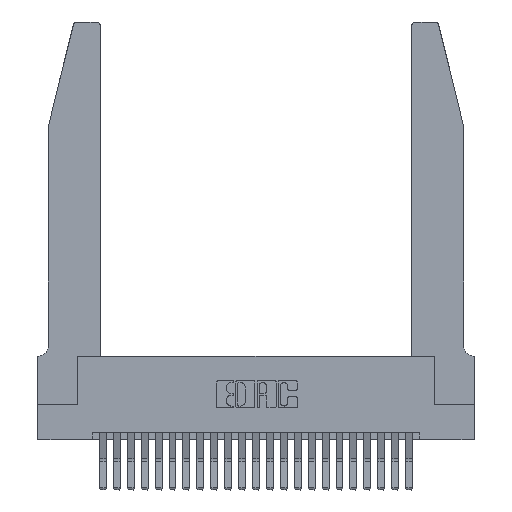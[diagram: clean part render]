
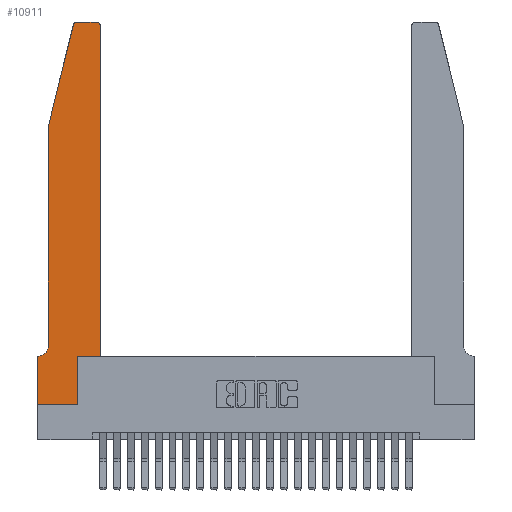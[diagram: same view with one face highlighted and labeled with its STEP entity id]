
A CAD part, top view. The second image highlights one B-rep face of the part: STEP entity #10911.
In plain terms, the highlighted planar face has unit normal (0, 0, 1).
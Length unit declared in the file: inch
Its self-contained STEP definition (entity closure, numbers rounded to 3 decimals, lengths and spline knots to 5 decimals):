
#15 = VECTOR ( 'NONE', #15309, 39.37008 ) ;
#550 = CARTESIAN_POINT ( 'NONE',  ( 0., 0., 0.37 ) ) ;
#933 = CARTESIAN_POINT ( 'NONE',  ( 0.0055, 0.35, 0.37 ) ) ;
#1262 = EDGE_CURVE ( 'NONE', #23223, #23100, #10198, .T. ) ;
#1471 = EDGE_LOOP ( 'NONE', ( #11044, #24769, #20503, #25360, #15903, #8886, #11153, #18814, #14873, #16694, #4052, #3981 ) ) ;
#1908 = EDGE_CURVE ( 'NONE', #11073, #17594, #23082, .T. ) ;
#2153 = VERTEX_POINT ( 'NONE', #11108 ) ;
#2604 = CARTESIAN_POINT ( 'NONE',  ( 0.284, 2.75, 0.37 ) ) ;
#2974 = VECTOR ( 'NONE', #14906, 39.37008 ) ;
#3108 = CARTESIAN_POINT ( 'NONE',  ( 0.0055, 0.42, 0.37 ) ) ;
#3163 = EDGE_CURVE ( 'NONE', #10190, #9971, #12925, .T. ) ;
#3170 = CIRCLE ( 'NONE', #18161, 0.03 ) ;
#3363 = CARTESIAN_POINT ( 'NONE',  ( 0.2865, 0.35, 0.37 ) ) ;
#3608 = EDGE_CURVE ( 'NONE', #23711, #13043, #4282, .T. ) ;
#3981 = ORIENTED_EDGE ( 'NONE', *, *, #11979, .T. ) ;
#4021 = DIRECTION ( 'NONE',  ( 0., -1., 0. ) ) ;
#4052 = ORIENTED_EDGE ( 'NONE', *, *, #1262, .T. ) ;
#4282 = LINE ( 'NONE', #23813, #11672 ) ;
#4654 = DIRECTION ( 'NONE',  ( 1., 0., 0. ) ) ;
#4776 = LINE ( 'NONE', #5056, #5112 ) ;
#4960 = CARTESIAN_POINT ( 'NONE',  ( 0.0755, 2., 0.37 ) ) ;
#5056 = CARTESIAN_POINT ( 'NONE',  ( 0.0755, 2., 0.37 ) ) ;
#5112 = VECTOR ( 'NONE', #18942, 39.37008 ) ;
#5397 = CARTESIAN_POINT ( 'NONE',  ( 0.284, 2.72, 0.37 ) ) ;
#5557 = CARTESIAN_POINT ( 'NONE',  ( 0., 0.35, 0.37 ) ) ;
#5687 = DIRECTION ( 'NONE',  ( 0., 1., 0. ) ) ;
#6547 = CARTESIAN_POINT ( 'NONE',  ( 0.4205, 2.72, 0.37 ) ) ;
#7175 = DIRECTION ( 'NONE',  ( 1., 0., 0. ) ) ;
#7464 = VECTOR ( 'NONE', #9497, 39.37008 ) ;
#8459 = DIRECTION ( 'NONE',  ( 1., 0., 0. ) ) ;
#8886 = ORIENTED_EDGE ( 'NONE', *, *, #1908, .T. ) ;
#9270 = DIRECTION ( 'NONE',  ( 0., 0., 1. ) ) ;
#9497 = DIRECTION ( 'NONE',  ( -1., 0., 0. ) ) ;
#9725 = CARTESIAN_POINT ( 'NONE',  ( 0.2865, 0.35, 0.37 ) ) ;
#9971 = VERTEX_POINT ( 'NONE', #2604 ) ;
#10190 = VERTEX_POINT ( 'NONE', #12941 ) ;
#10198 = LINE ( 'NONE', #10573, #15727 ) ;
#10573 = CARTESIAN_POINT ( 'NONE',  ( 0.4505, 0.35, 0.37 ) ) ;
#10820 = CARTESIAN_POINT ( 'NONE',  ( 0.4505, 0.35, 0.37 ) ) ;
#10904 = PLANE ( 'NONE',  #17168 ) ;
#10911 = ADVANCED_FACE ( 'NONE', ( #11515 ), #10904, .T. ) ;
#11044 = ORIENTED_EDGE ( 'NONE', *, *, #3163, .T. ) ;
#11073 = VERTEX_POINT ( 'NONE', #933 ) ;
#11108 = CARTESIAN_POINT ( 'NONE',  ( 0.25487, 2.72718, 0.37 ) ) ;
#11153 = ORIENTED_EDGE ( 'NONE', *, *, #12731, .T. ) ;
#11278 = CIRCLE ( 'NONE', #12000, 0.07 ) ;
#11515 = FACE_OUTER_BOUND ( 'NONE', #1471, .T. ) ;
#11672 = VECTOR ( 'NONE', #4021, 39.37008 ) ;
#11979 = EDGE_CURVE ( 'NONE', #23100, #10190, #3170, .T. ) ;
#12000 = AXIS2_PLACEMENT_3D ( 'NONE', #3108, #18172, #20139 ) ;
#12214 = VERTEX_POINT ( 'NONE', #20488 ) ;
#12731 = EDGE_CURVE ( 'NONE', #17594, #12214, #21824, .T. ) ;
#12816 = EDGE_CURVE ( 'NONE', #21832, #23223, #19686, .T. ) ;
#12925 = LINE ( 'NONE', #17360, #15 ) ;
#12941 = CARTESIAN_POINT ( 'NONE',  ( 0.4205, 2.75, 0.37 ) ) ;
#13043 = VERTEX_POINT ( 'NONE', #23539 ) ;
#13583 = CARTESIAN_POINT ( 'NONE',  ( 0., 0.35, 0.37 ) ) ;
#14128 = VECTOR ( 'NONE', #5687, 39.37008 ) ;
#14820 = CARTESIAN_POINT ( 'NONE',  ( 0.0755, 0.35, 0.37 ) ) ;
#14873 = ORIENTED_EDGE ( 'NONE', *, *, #14884, .T. ) ;
#14884 = EDGE_CURVE ( 'NONE', #17351, #21832, #16625, .T. ) ;
#14906 = DIRECTION ( 'NONE',  ( 1., 0., 0. ) ) ;
#14942 = DIRECTION ( 'NONE',  ( 0., 0., 1. ) ) ;
#15095 = DIRECTION ( 'NONE',  ( 1., 0., 0. ) ) ;
#15309 = DIRECTION ( 'NONE',  ( -1., 0., 0. ) ) ;
#15727 = VECTOR ( 'NONE', #18652, 39.37008 ) ;
#15903 = ORIENTED_EDGE ( 'NONE', *, *, #19192, .T. ) ;
#16625 = LINE ( 'NONE', #3363, #14128 ) ;
#16694 = ORIENTED_EDGE ( 'NONE', *, *, #12816, .T. ) ;
#17168 = AXIS2_PLACEMENT_3D ( 'NONE', #5557, #9270, #15095 ) ;
#17351 = VERTEX_POINT ( 'NONE', #20990 ) ;
#17360 = CARTESIAN_POINT ( 'NONE',  ( 0.2605, 2.75, 0.37 ) ) ;
#17594 = VERTEX_POINT ( 'NONE', #13583 ) ;
#18161 = AXIS2_PLACEMENT_3D ( 'NONE', #6547, #22230, #4654 ) ;
#18172 = DIRECTION ( 'NONE',  ( 0., 0., -1. ) ) ;
#18652 = DIRECTION ( 'NONE',  ( 0., 1., 0. ) ) ;
#18814 = ORIENTED_EDGE ( 'NONE', *, *, #23839, .T. ) ;
#18942 = DIRECTION ( 'NONE',  ( -0.239, -0.971, 0. ) ) ;
#19062 = DIRECTION ( 'NONE',  ( 0., -1., 0. ) ) ;
#19087 = VECTOR ( 'NONE', #19062, 39.37008 ) ;
#19114 = AXIS2_PLACEMENT_3D ( 'NONE', #5397, #14942, #7175 ) ;
#19192 = EDGE_CURVE ( 'NONE', #13043, #11073, #11278, .T. ) ;
#19686 = LINE ( 'NONE', #21830, #20597 ) ;
#20052 = CARTESIAN_POINT ( 'NONE',  ( 0.4505, 2.72, 0.37 ) ) ;
#20139 = DIRECTION ( 'NONE',  ( -1., 0., 0. ) ) ;
#20488 = CARTESIAN_POINT ( 'NONE',  ( 0., 0., 0.37 ) ) ;
#20503 = ORIENTED_EDGE ( 'NONE', *, *, #24466, .T. ) ;
#20522 = EDGE_CURVE ( 'NONE', #9971, #2153, #22349, .T. ) ;
#20597 = VECTOR ( 'NONE', #8459, 39.37008 ) ;
#20990 = CARTESIAN_POINT ( 'NONE',  ( 0.2865, 0., 0.37 ) ) ;
#21824 = LINE ( 'NONE', #550, #19087 ) ;
#21830 = CARTESIAN_POINT ( 'NONE',  ( 0.4505, 0.35, 0.37 ) ) ;
#21832 = VERTEX_POINT ( 'NONE', #9725 ) ;
#22230 = DIRECTION ( 'NONE',  ( 0., 0., 1. ) ) ;
#22349 = CIRCLE ( 'NONE', #19114, 0.03 ) ;
#23059 = CARTESIAN_POINT ( 'NONE',  ( 0., 0., 0.37 ) ) ;
#23082 = LINE ( 'NONE', #14820, #7464 ) ;
#23100 = VERTEX_POINT ( 'NONE', #20052 ) ;
#23223 = VERTEX_POINT ( 'NONE', #10820 ) ;
#23539 = CARTESIAN_POINT ( 'NONE',  ( 0.0755, 0.42, 0.37 ) ) ;
#23711 = VERTEX_POINT ( 'NONE', #4960 ) ;
#23813 = CARTESIAN_POINT ( 'NONE',  ( 0.0755, 2., 0.37 ) ) ;
#23820 = LINE ( 'NONE', #23059, #2974 ) ;
#23839 = EDGE_CURVE ( 'NONE', #12214, #17351, #23820, .T. ) ;
#24466 = EDGE_CURVE ( 'NONE', #2153, #23711, #4776, .T. ) ;
#24769 = ORIENTED_EDGE ( 'NONE', *, *, #20522, .T. ) ;
#25360 = ORIENTED_EDGE ( 'NONE', *, *, #3608, .T. ) ;
